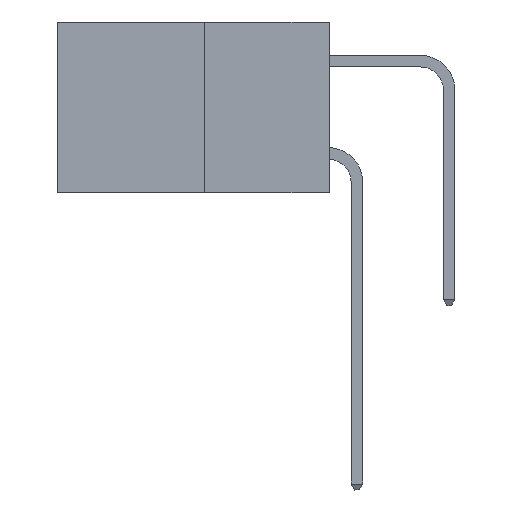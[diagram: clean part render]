
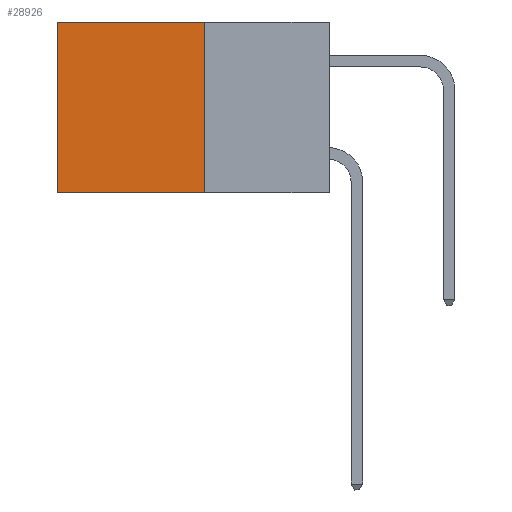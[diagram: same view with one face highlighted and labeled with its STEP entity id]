
A CAD part, left-side view. The second image highlights one B-rep face of the part: STEP entity #28926.
In plain terms, the highlighted planar face has unit normal (-1, 0, 0).
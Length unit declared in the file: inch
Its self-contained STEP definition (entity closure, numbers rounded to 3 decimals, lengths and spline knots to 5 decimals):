
#1855 = CARTESIAN_POINT ( 'NONE',  ( 0.277, 0.27, 0. ) ) ;
#2292 = DIRECTION ( 'NONE',  ( 0., 1., 0. ) ) ;
#2430 = CARTESIAN_POINT ( 'NONE',  ( 0.277, 0.27, -0.37 ) ) ;
#4068 = ORIENTED_EDGE ( 'NONE', *, *, #7150, .F. ) ;
#4624 = CARTESIAN_POINT ( 'NONE',  ( 0.277, 0.27, -0.37 ) ) ;
#4718 = LINE ( 'NONE', #28009, #18524 ) ;
#5250 = EDGE_CURVE ( 'NONE', #22987, #18754, #6415, .T. ) ;
#5747 = EDGE_CURVE ( 'NONE', #18754, #20489, #4718, .T. ) ;
#6415 = LINE ( 'NONE', #9216, #19366 ) ;
#6585 = VECTOR ( 'NONE', #30301, 39.37008 ) ;
#7150 = EDGE_CURVE ( 'NONE', #19606, #20489, #31201, .T. ) ;
#8217 = LINE ( 'NONE', #4624, #6585 ) ;
#9216 = CARTESIAN_POINT ( 'NONE',  ( 0.277, 0.27, 0. ) ) ;
#9435 = EDGE_CURVE ( 'NONE', #22987, #19606, #8217, .T. ) ;
#9846 = DIRECTION ( 'NONE',  ( 0., 1., 0. ) ) ;
#10389 = VECTOR ( 'NONE', #2292, 39.37008 ) ;
#11889 = CARTESIAN_POINT ( 'NONE',  ( 0.277, 0.27, -0.37 ) ) ;
#12814 = AXIS2_PLACEMENT_3D ( 'NONE', #11889, #29802, #14451 ) ;
#14451 = DIRECTION ( 'NONE',  ( 0., 0., -1. ) ) ;
#15664 = CARTESIAN_POINT ( 'NONE',  ( 0.277, 0.59, -0.37 ) ) ;
#16350 = EDGE_LOOP ( 'NONE', ( #18827, #4068, #21847, #32231 ) ) ;
#18524 = VECTOR ( 'NONE', #28157, 39.37008 ) ;
#18754 = VERTEX_POINT ( 'NONE', #31676 ) ;
#18827 = ORIENTED_EDGE ( 'NONE', *, *, #5747, .T. ) ;
#19366 = VECTOR ( 'NONE', #9846, 39.37008 ) ;
#19606 = VERTEX_POINT ( 'NONE', #20147 ) ;
#20147 = CARTESIAN_POINT ( 'NONE',  ( 0.277, 0.27, -0.37 ) ) ;
#20489 = VERTEX_POINT ( 'NONE', #15664 ) ;
#21847 = ORIENTED_EDGE ( 'NONE', *, *, #9435, .F. ) ;
#22987 = VERTEX_POINT ( 'NONE', #1855 ) ;
#26198 = FACE_OUTER_BOUND ( 'NONE', #16350, .T. ) ;
#27237 = PLANE ( 'NONE',  #12814 ) ;
#28009 = CARTESIAN_POINT ( 'NONE',  ( 0.277, 0.59, -0.37 ) ) ;
#28157 = DIRECTION ( 'NONE',  ( 0., 0., -1. ) ) ;
#28926 = ADVANCED_FACE ( 'NONE', ( #26198 ), #27237, .F. ) ;
#29802 = DIRECTION ( 'NONE',  ( 1., 0., 0. ) ) ;
#30301 = DIRECTION ( 'NONE',  ( 0., 0., -1. ) ) ;
#31201 = LINE ( 'NONE', #2430, #10389 ) ;
#31676 = CARTESIAN_POINT ( 'NONE',  ( 0.277, 0.59, 0. ) ) ;
#32231 = ORIENTED_EDGE ( 'NONE', *, *, #5250, .T. ) ;
